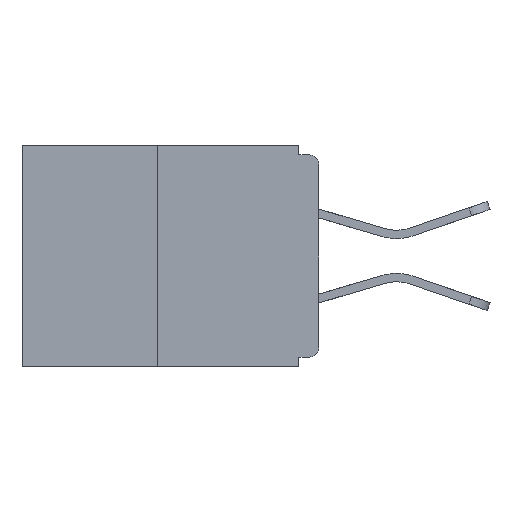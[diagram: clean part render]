
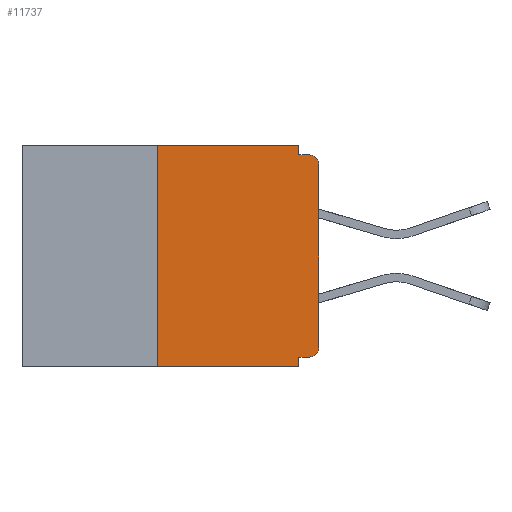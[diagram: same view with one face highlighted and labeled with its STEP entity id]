
A CAD part, left-side view. The second image highlights one B-rep face of the part: STEP entity #11737.
In plain terms, the highlighted planar face has unit normal (-1, 0, 0).
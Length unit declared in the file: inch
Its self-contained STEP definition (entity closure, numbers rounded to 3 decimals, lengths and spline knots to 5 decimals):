
#1 = DIRECTION ( 'NONE',  ( 0., 0., -1. ) ) ;
#24 = ORIENTED_EDGE ( 'NONE', *, *, #9025, .T. ) ;
#50 = VERTEX_POINT ( 'NONE', #15309 ) ;
#55 = CARTESIAN_POINT ( 'NONE',  ( 0., 0.25, 0. ) ) ;
#63 = EDGE_LOOP ( 'NONE', ( #9327, #14986, #3789, #4899, #901, #11981, #24, #10499, #10798, #10912 ) ) ;
#106 = VERTEX_POINT ( 'NONE', #4637 ) ;
#373 = VECTOR ( 'NONE', #2746, 39.37008 ) ;
#858 = CIRCLE ( 'NONE', #3341, 0.015 ) ;
#901 = ORIENTED_EDGE ( 'NONE', *, *, #10876, .F. ) ;
#1679 = VERTEX_POINT ( 'NONE', #3057 ) ;
#1736 = CARTESIAN_POINT ( 'NONE',  ( 0., 0.015, -0.015 ) ) ;
#1887 = DIRECTION ( 'NONE',  ( 0., 0., -1. ) ) ;
#2099 = LINE ( 'NONE', #13060, #11012 ) ;
#2376 = DIRECTION ( 'NONE',  ( 0., 0., 1. ) ) ;
#2457 = AXIS2_PLACEMENT_3D ( 'NONE', #11442, #9012, #1887 ) ;
#2589 = CARTESIAN_POINT ( 'NONE',  ( 0., 0.031, -0.343 ) ) ;
#2678 = EDGE_CURVE ( 'NONE', #8800, #106, #14182, .T. ) ;
#2746 = DIRECTION ( 'NONE',  ( 0., 0., -1. ) ) ;
#2873 = VERTEX_POINT ( 'NONE', #8956 ) ;
#3057 = CARTESIAN_POINT ( 'NONE',  ( 0., 0.25, -0.343 ) ) ;
#3135 = FACE_OUTER_BOUND ( 'NONE', #63, .T. ) ;
#3262 = VECTOR ( 'NONE', #4798, 39.37008 ) ;
#3341 = AXIS2_PLACEMENT_3D ( 'NONE', #5807, #11871, #1 ) ;
#3372 = VERTEX_POINT ( 'NONE', #6578 ) ;
#3376 = EDGE_CURVE ( 'NONE', #3372, #5265, #10807, .T. ) ;
#3789 = ORIENTED_EDGE ( 'NONE', *, *, #6389, .T. ) ;
#4069 = EDGE_CURVE ( 'NONE', #1679, #5286, #6288, .T. ) ;
#4637 = CARTESIAN_POINT ( 'NONE',  ( 0., 0.031, -0.015 ) ) ;
#4798 = DIRECTION ( 'NONE',  ( 0., -1., 0. ) ) ;
#4899 = ORIENTED_EDGE ( 'NONE', *, *, #10987, .F. ) ;
#5265 = VERTEX_POINT ( 'NONE', #13079 ) ;
#5286 = VERTEX_POINT ( 'NONE', #55 ) ;
#5506 = CARTESIAN_POINT ( 'NONE',  ( 0., 0.031, 0. ) ) ;
#5701 = CARTESIAN_POINT ( 'NONE',  ( 0., 0.46, 0. ) ) ;
#5807 = CARTESIAN_POINT ( 'NONE',  ( 0., 0.015, -0.03 ) ) ;
#6013 = VECTOR ( 'NONE', #13861, 39.37008 ) ;
#6117 = CARTESIAN_POINT ( 'NONE',  ( 0., 0.031, 0. ) ) ;
#6240 = VERTEX_POINT ( 'NONE', #9764 ) ;
#6288 = LINE ( 'NONE', #9570, #11719 ) ;
#6389 = EDGE_CURVE ( 'NONE', #1679, #2873, #14233, .T. ) ;
#6578 = CARTESIAN_POINT ( 'NONE',  ( 0., 0.015, -0.328 ) ) ;
#7707 = AXIS2_PLACEMENT_3D ( 'NONE', #5701, #15070, #8175 ) ;
#8125 = EDGE_CURVE ( 'NONE', #5286, #8800, #10676, .T. ) ;
#8175 = DIRECTION ( 'NONE',  ( 0., 0., -1. ) ) ;
#8256 = EDGE_CURVE ( 'NONE', #6240, #8746, #858, .T. ) ;
#8746 = VERTEX_POINT ( 'NONE', #1736 ) ;
#8800 = VERTEX_POINT ( 'NONE', #5506 ) ;
#8956 = CARTESIAN_POINT ( 'NONE',  ( 0., 0.031, -0.343 ) ) ;
#9012 = DIRECTION ( 'NONE',  ( -1., 0., 0. ) ) ;
#9025 = EDGE_CURVE ( 'NONE', #5265, #6240, #2099, .T. ) ;
#9306 = LINE ( 'NONE', #2589, #373 ) ;
#9327 = ORIENTED_EDGE ( 'NONE', *, *, #8125, .F. ) ;
#9570 = CARTESIAN_POINT ( 'NONE',  ( 0., 0.25, 0. ) ) ;
#9637 = DIRECTION ( 'NONE',  ( 0., 0., 1. ) ) ;
#9764 = CARTESIAN_POINT ( 'NONE',  ( 0., 0., -0.03 ) ) ;
#10176 = DIRECTION ( 'NONE',  ( 0., -1., 0. ) ) ;
#10446 = EDGE_CURVE ( 'NONE', #106, #8746, #13568, .T. ) ;
#10499 = ORIENTED_EDGE ( 'NONE', *, *, #8256, .T. ) ;
#10515 = PLANE ( 'NONE',  #7707 ) ;
#10600 = CARTESIAN_POINT ( 'NONE',  ( 0., 0., -0.328 ) ) ;
#10676 = LINE ( 'NONE', #10792, #3262 ) ;
#10792 = CARTESIAN_POINT ( 'NONE',  ( 0., 0.46, 0. ) ) ;
#10798 = ORIENTED_EDGE ( 'NONE', *, *, #10446, .F. ) ;
#10807 = CIRCLE ( 'NONE', #2457, 0.015 ) ;
#10876 = EDGE_CURVE ( 'NONE', #3372, #50, #11883, .T. ) ;
#10912 = ORIENTED_EDGE ( 'NONE', *, *, #2678, .F. ) ;
#10987 = EDGE_CURVE ( 'NONE', #50, #2873, #9306, .T. ) ;
#11012 = VECTOR ( 'NONE', #9637, 39.37008 ) ;
#11442 = CARTESIAN_POINT ( 'NONE',  ( 0., 0.015, -0.313 ) ) ;
#11517 = CARTESIAN_POINT ( 'NONE',  ( 0., 0.46, -0.343 ) ) ;
#11719 = VECTOR ( 'NONE', #2376, 39.37008 ) ;
#11737 = ADVANCED_FACE ( 'NONE', ( #3135 ), #10515, .F. ) ;
#11747 = DIRECTION ( 'NONE',  ( 0., 1., 0. ) ) ;
#11864 = DIRECTION ( 'NONE',  ( 0., 0., -1. ) ) ;
#11871 = DIRECTION ( 'NONE',  ( -1., 0., 0. ) ) ;
#11883 = LINE ( 'NONE', #10600, #12081 ) ;
#11981 = ORIENTED_EDGE ( 'NONE', *, *, #3376, .T. ) ;
#12081 = VECTOR ( 'NONE', #11747, 39.37008 ) ;
#13028 = VECTOR ( 'NONE', #10176, 39.37008 ) ;
#13060 = CARTESIAN_POINT ( 'NONE',  ( 0., 0., 0. ) ) ;
#13079 = CARTESIAN_POINT ( 'NONE',  ( 0., 0., -0.313 ) ) ;
#13568 = LINE ( 'NONE', #14921, #13028 ) ;
#13861 = DIRECTION ( 'NONE',  ( 0., -1., 0. ) ) ;
#13984 = VECTOR ( 'NONE', #11864, 39.37008 ) ;
#14182 = LINE ( 'NONE', #6117, #13984 ) ;
#14233 = LINE ( 'NONE', #11517, #6013 ) ;
#14921 = CARTESIAN_POINT ( 'NONE',  ( 0., 0., -0.015 ) ) ;
#14986 = ORIENTED_EDGE ( 'NONE', *, *, #4069, .F. ) ;
#15070 = DIRECTION ( 'NONE',  ( 1., 0., 0. ) ) ;
#15309 = CARTESIAN_POINT ( 'NONE',  ( 0., 0.031, -0.328 ) ) ;
